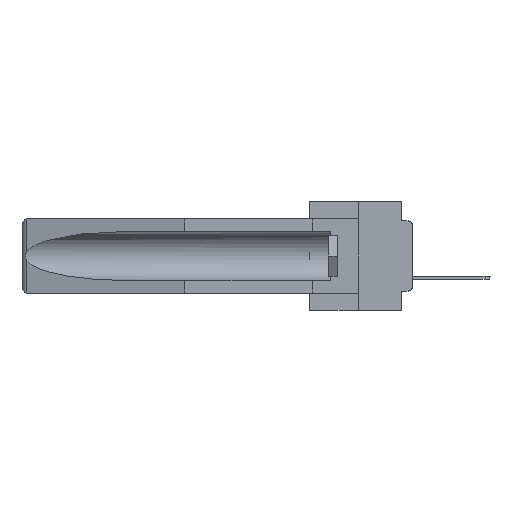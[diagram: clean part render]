
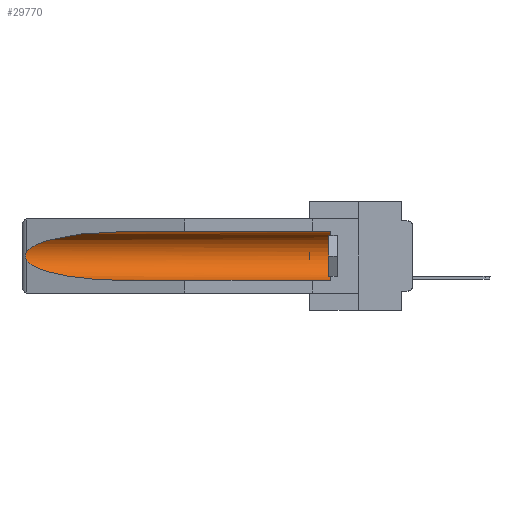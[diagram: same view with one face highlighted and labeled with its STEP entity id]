
A CAD part, left-side view. The second image highlights one B-rep face of the part: STEP entity #29770.
In plain terms, the highlighted cylindrical face has radius 2.857 mm (diameter 5.715 mm), a partial arc.
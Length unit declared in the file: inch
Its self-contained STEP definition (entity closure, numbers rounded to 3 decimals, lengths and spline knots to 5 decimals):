
#1556 = EDGE_CURVE ( 'NONE', #16332, #8451, #6557, .T. ) ;
#1868 =( BOUNDED_CURVE ( )  B_SPLINE_CURVE ( 3, ( #21173, #21757, #33868, #33284 ),
 .UNSPECIFIED., .F., .F. ) 
 B_SPLINE_CURVE_WITH_KNOTS ( ( 4, 4 ),
 ( 0.1948, 1.5708 ),
 .UNSPECIFIED. ) 
 CURVE ( )  GEOMETRIC_REPRESENTATION_ITEM ( )  RATIONAL_B_SPLINE_CURVE ( ( 1., 0.848, 0.848, 1. ) ) 
 REPRESENTATION_ITEM ( '' )  );
#1953 = VERTEX_POINT ( 'NONE', #18948 ) ;
#2081 = CARTESIAN_POINT ( 'NONE',  ( 0.26597, 1.5296, -0.19026 ) ) ;
#2135 = CARTESIAN_POINT ( 'NONE',  ( 0.26537, 1.52718, -0.14972 ) ) ;
#3812 = CARTESIAN_POINT ( 'NONE',  ( 0.155, 1.07973, -0.059 ) ) ;
#4082 = VECTOR ( 'NONE', #25090, 39.37008 ) ;
#5122 = CARTESIAN_POINT ( 'NONE',  ( 0.26654, 1.53092, -0.15636 ) ) ;
#6374 = ORIENTED_EDGE ( 'NONE', *, *, #15114, .T. ) ;
#6557 = LINE ( 'NONE', #30753, #4082 ) ;
#7795 = VERTEX_POINT ( 'NONE', #38602 ) ;
#8451 = VERTEX_POINT ( 'NONE', #3812 ) ;
#10523 = CARTESIAN_POINT ( 'NONE',  ( 0.155, -0.30754, -0.1715 ) ) ;
#11137 = DIRECTION ( 'NONE',  ( 0., 1., 0. ) ) ;
#12881 = EDGE_LOOP ( 'NONE', ( #38600, #26307, #24157, #25881, #6374, #34800 ) ) ;
#13070 = LINE ( 'NONE', #22940, #25684 ) ;
#13889 = DIRECTION ( 'NONE',  ( 0., -1., 0. ) ) ;
#14388 = CARTESIAN_POINT ( 'NONE',  ( 0.26537, 1.52718, -0.19328 ) ) ;
#15114 = EDGE_CURVE ( 'NONE', #1953, #16332, #29782, .T. ) ;
#16332 = VERTEX_POINT ( 'NONE', #37363 ) ;
#17402 = CARTESIAN_POINT ( 'NONE',  ( 0.2673, 1.53269, -0.17917 ) ) ;
#18948 = CARTESIAN_POINT ( 'NONE',  ( 0.155, 0.126, -0.284 ) ) ;
#19314 = DIRECTION ( 'NONE',  ( 0., 1., 0. ) ) ;
#20443 = CARTESIAN_POINT ( 'NONE',  ( 0.155, 1.07973, -0.284 ) ) ;
#20531 = DIRECTION ( 'NONE',  ( 0., 0., 1. ) ) ;
#21173 = CARTESIAN_POINT ( 'NONE',  ( 0.26537, 1.52718, -0.19328 ) ) ;
#21757 = CARTESIAN_POINT ( 'NONE',  ( 0.25451, 1.48313, -0.24835 ) ) ;
#22940 = CARTESIAN_POINT ( 'NONE',  ( 0.155, -0.30754, -0.284 ) ) ;
#23274 = EDGE_CURVE ( 'NONE', #1953, #28205, #13070, .T. ) ;
#23386 = VERTEX_POINT ( 'NONE', #29576 ) ;
#23460 = CARTESIAN_POINT ( 'NONE',  ( 0.26537, 1.52718, -0.14972 ) ) ;
#24061 = CARTESIAN_POINT ( 'NONE',  ( 0.2673, 1.5327, -0.16383 ) ) ;
#24157 = ORIENTED_EDGE ( 'NONE', *, *, #32810, .T. ) ;
#24362 = AXIS2_PLACEMENT_3D ( 'NONE', #10523, #11137, #37967 ) ;
#25090 = DIRECTION ( 'NONE',  ( 0., 1., 0. ) ) ;
#25684 = VECTOR ( 'NONE', #19314, 39.37008 ) ;
#25881 = ORIENTED_EDGE ( 'NONE', *, *, #23274, .F. ) ;
#26307 = ORIENTED_EDGE ( 'NONE', *, *, #33554, .T. ) ;
#26939 = CARTESIAN_POINT ( 'NONE',  ( 0.155, 1.07973, -0.059 ) ) ;
#28205 = VERTEX_POINT ( 'NONE', #20443 ) ;
#29152 = AXIS2_PLACEMENT_3D ( 'NONE', #35468, #13889, #20531 ) ;
#29576 = CARTESIAN_POINT ( 'NONE',  ( 0.26537, 1.52718, -0.14972 ) ) ;
#29702 = CARTESIAN_POINT ( 'NONE',  ( 0.26655, 1.53094, -0.18657 ) ) ;
#29770 = ADVANCED_FACE ( 'NONE', ( #35133 ), #38769, .F. ) ;
#29782 = CIRCLE ( 'NONE', #29152, 0.1125 ) ;
#29895 = CARTESIAN_POINT ( 'NONE',  ( 0.26597, 1.52961, -0.15275 ) ) ;
#30753 = CARTESIAN_POINT ( 'NONE',  ( 0.155, -0.30754, -0.059 ) ) ;
#32062 = B_SPLINE_CURVE_WITH_KNOTS ( 'NONE', 3,
 ( #23460, #29895, #5122, #24061, #39401, #33139, #17402, #29702, #2081, #14388 ),
 .UNSPECIFIED., .F., .F.,
 ( 4, 2, 2, 2, 4 ),
 ( 0., 0.00029, 0.00058, 0.00087, 0.00117 ),
 .UNSPECIFIED. ) ;
#32801 = CARTESIAN_POINT ( 'NONE',  ( 0.21114, 1.30732, -0.059 ) ) ;
#32810 = EDGE_CURVE ( 'NONE', #7795, #28205, #1868, .T. ) ;
#33139 = CARTESIAN_POINT ( 'NONE',  ( 0.2675, 1.53308, -0.17534 ) ) ;
#33284 = CARTESIAN_POINT ( 'NONE',  ( 0.155, 1.07973, -0.284 ) ) ;
#33554 = EDGE_CURVE ( 'NONE', #23386, #7795, #32062, .T. ) ;
#33868 = CARTESIAN_POINT ( 'NONE',  ( 0.21114, 1.30732, -0.284 ) ) ;
#34384 =( BOUNDED_CURVE ( )  B_SPLINE_CURVE ( 3, ( #26939, #32801, #36018, #2135 ),
 .UNSPECIFIED., .F., .F. ) 
 B_SPLINE_CURVE_WITH_KNOTS ( ( 4, 4 ),
 ( 4.71239, 6.08839 ),
 .UNSPECIFIED. ) 
 CURVE ( )  GEOMETRIC_REPRESENTATION_ITEM ( )  RATIONAL_B_SPLINE_CURVE ( ( 1., 0.848, 0.848, 1. ) ) 
 REPRESENTATION_ITEM ( '' )  );
#34800 = ORIENTED_EDGE ( 'NONE', *, *, #1556, .T. ) ;
#35133 = FACE_OUTER_BOUND ( 'NONE', #12881, .T. ) ;
#35314 = EDGE_CURVE ( 'NONE', #8451, #23386, #34384, .T. ) ;
#35468 = CARTESIAN_POINT ( 'NONE',  ( 0.155, 0.126, -0.1715 ) ) ;
#36018 = CARTESIAN_POINT ( 'NONE',  ( 0.25451, 1.48313, -0.09465 ) ) ;
#37363 = CARTESIAN_POINT ( 'NONE',  ( 0.155, 0.126, -0.059 ) ) ;
#37967 = DIRECTION ( 'NONE',  ( 0., 0., 1. ) ) ;
#38600 = ORIENTED_EDGE ( 'NONE', *, *, #35314, .T. ) ;
#38602 = CARTESIAN_POINT ( 'NONE',  ( 0.26537, 1.52718, -0.19328 ) ) ;
#38769 = CYLINDRICAL_SURFACE ( 'NONE', #24362, 0.1125 ) ;
#39401 = CARTESIAN_POINT ( 'NONE',  ( 0.2675, 1.53308, -0.16763 ) ) ;
